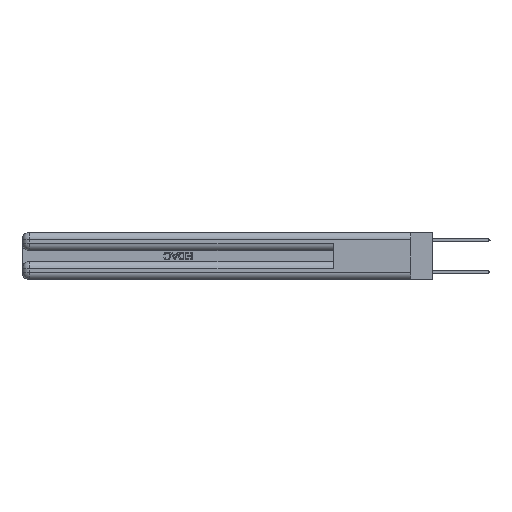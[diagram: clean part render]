
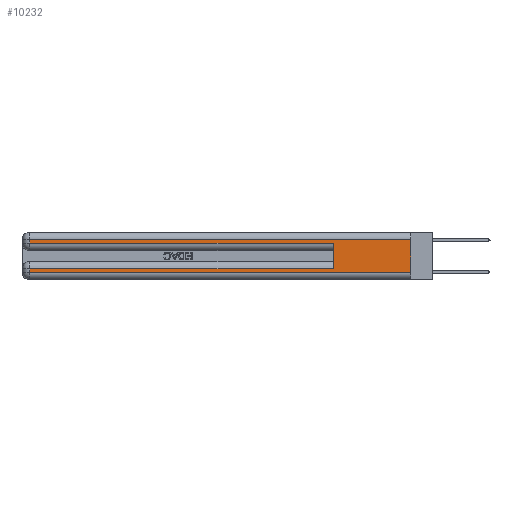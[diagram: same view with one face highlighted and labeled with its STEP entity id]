
A CAD part, left-side view. The second image highlights one B-rep face of the part: STEP entity #10232.
In plain terms, the highlighted planar face has unit normal (-1, 0, 0).
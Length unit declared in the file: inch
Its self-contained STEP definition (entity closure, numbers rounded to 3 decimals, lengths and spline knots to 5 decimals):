
#623 = CARTESIAN_POINT ( 'NONE',  ( 0., 0.6, 0.285 ) ) ;
#1055 = FACE_OUTER_BOUND ( 'NONE', #4014, .T. ) ;
#1336 = CARTESIAN_POINT ( 'NONE',  ( 0., 0., 0.31 ) ) ;
#1669 = EDGE_CURVE ( 'NONE', #15549, #18901, #19831, .T. ) ;
#2334 = ORIENTED_EDGE ( 'NONE', *, *, #14169, .T. ) ;
#3235 = EDGE_CURVE ( 'NONE', #19497, #26161, #14407, .T. ) ;
#3728 = CARTESIAN_POINT ( 'NONE',  ( 0., 0., 0.37 ) ) ;
#4014 = EDGE_LOOP ( 'NONE', ( #15367, #2334, #29586, #16734, #31900, #23918, #18109, #5466 ) ) ;
#4241 = EDGE_CURVE ( 'NONE', #26161, #19588, #33213, .T. ) ;
#4714 = CARTESIAN_POINT ( 'NONE',  ( 0., 2.94, 0.285 ) ) ;
#5182 = CARTESIAN_POINT ( 'NONE',  ( 0., 0.6, 0.145 ) ) ;
#5466 = ORIENTED_EDGE ( 'NONE', *, *, #31265, .T. ) ;
#6227 = DIRECTION ( 'NONE',  ( 0., 0., -1. ) ) ;
#7387 = VERTEX_POINT ( 'NONE', #623 ) ;
#7595 = CARTESIAN_POINT ( 'NONE',  ( 0., 0., 0.06 ) ) ;
#7650 = CARTESIAN_POINT ( 'NONE',  ( 0., 0., 0.085 ) ) ;
#8031 = DIRECTION ( 'NONE',  ( 0., 0., -1. ) ) ;
#8354 = CARTESIAN_POINT ( 'NONE',  ( 0., 2.94, 0.06 ) ) ;
#8561 = LINE ( 'NONE', #12270, #29111 ) ;
#9115 = LINE ( 'NONE', #5182, #29332 ) ;
#9157 = DIRECTION ( 'NONE',  ( 1., 0., 0. ) ) ;
#9176 = CARTESIAN_POINT ( 'NONE',  ( 0., 2.94, 0.31 ) ) ;
#10232 = ADVANCED_FACE ( 'NONE', ( #1055 ), #33203, .F. ) ;
#10382 = DIRECTION ( 'NONE',  ( 0., 1., 0. ) ) ;
#10992 = VECTOR ( 'NONE', #17497, 39.37008 ) ;
#11661 = CARTESIAN_POINT ( 'NONE',  ( 0., 2.94, 0.37 ) ) ;
#11819 = VECTOR ( 'NONE', #8031, 39.37008 ) ;
#11867 = LINE ( 'NONE', #21849, #25319 ) ;
#12270 = CARTESIAN_POINT ( 'NONE',  ( 0., 0., 0.285 ) ) ;
#12292 = LINE ( 'NONE', #7595, #32851 ) ;
#12355 = CARTESIAN_POINT ( 'NONE',  ( 0., 0., 0.31 ) ) ;
#13960 = EDGE_CURVE ( 'NONE', #15695, #24640, #11867, .T. ) ;
#14169 = EDGE_CURVE ( 'NONE', #15695, #15549, #19830, .T. ) ;
#14407 = LINE ( 'NONE', #7650, #28660 ) ;
#15367 = ORIENTED_EDGE ( 'NONE', *, *, #13960, .F. ) ;
#15549 = VERTEX_POINT ( 'NONE', #9176 ) ;
#15695 = VERTEX_POINT ( 'NONE', #12355 ) ;
#16734 = ORIENTED_EDGE ( 'NONE', *, *, #17045, .T. ) ;
#17045 = EDGE_CURVE ( 'NONE', #18901, #7387, #8561, .T. ) ;
#17497 = DIRECTION ( 'NONE',  ( 0., 1., 0. ) ) ;
#18109 = ORIENTED_EDGE ( 'NONE', *, *, #4241, .T. ) ;
#18437 = DIRECTION ( 'NONE',  ( 0., -1., 0. ) ) ;
#18901 = VERTEX_POINT ( 'NONE', #4714 ) ;
#19497 = VERTEX_POINT ( 'NONE', #34597 ) ;
#19588 = VERTEX_POINT ( 'NONE', #8354 ) ;
#19830 = LINE ( 'NONE', #1336, #10992 ) ;
#19831 = LINE ( 'NONE', #11661, #26114 ) ;
#20334 = CARTESIAN_POINT ( 'NONE',  ( 0., 0., 0.06 ) ) ;
#20825 = EDGE_CURVE ( 'NONE', #19497, #7387, #9115, .T. ) ;
#21547 = AXIS2_PLACEMENT_3D ( 'NONE', #3728, #9157, #27938 ) ;
#21849 = CARTESIAN_POINT ( 'NONE',  ( 0., 0., 0.37 ) ) ;
#23918 = ORIENTED_EDGE ( 'NONE', *, *, #3235, .T. ) ;
#24027 = DIRECTION ( 'NONE',  ( 0., 0., 1. ) ) ;
#24640 = VERTEX_POINT ( 'NONE', #20334 ) ;
#25319 = VECTOR ( 'NONE', #32633, 39.37008 ) ;
#26114 = VECTOR ( 'NONE', #6227, 39.37008 ) ;
#26161 = VERTEX_POINT ( 'NONE', #27493 ) ;
#26812 = CARTESIAN_POINT ( 'NONE',  ( 0., 2.94, 0.37 ) ) ;
#27493 = CARTESIAN_POINT ( 'NONE',  ( 0., 2.94, 0.085 ) ) ;
#27938 = DIRECTION ( 'NONE',  ( 0., 0., -1. ) ) ;
#28660 = VECTOR ( 'NONE', #10382, 39.37008 ) ;
#29111 = VECTOR ( 'NONE', #33714, 39.37008 ) ;
#29332 = VECTOR ( 'NONE', #24027, 39.37008 ) ;
#29586 = ORIENTED_EDGE ( 'NONE', *, *, #1669, .T. ) ;
#31265 = EDGE_CURVE ( 'NONE', #19588, #24640, #12292, .T. ) ;
#31900 = ORIENTED_EDGE ( 'NONE', *, *, #20825, .F. ) ;
#32633 = DIRECTION ( 'NONE',  ( 0., 0., -1. ) ) ;
#32851 = VECTOR ( 'NONE', #18437, 39.37008 ) ;
#33203 = PLANE ( 'NONE',  #21547 ) ;
#33213 = LINE ( 'NONE', #26812, #11819 ) ;
#33714 = DIRECTION ( 'NONE',  ( 0., -1., 0. ) ) ;
#34597 = CARTESIAN_POINT ( 'NONE',  ( 0., 0.6, 0.085 ) ) ;
